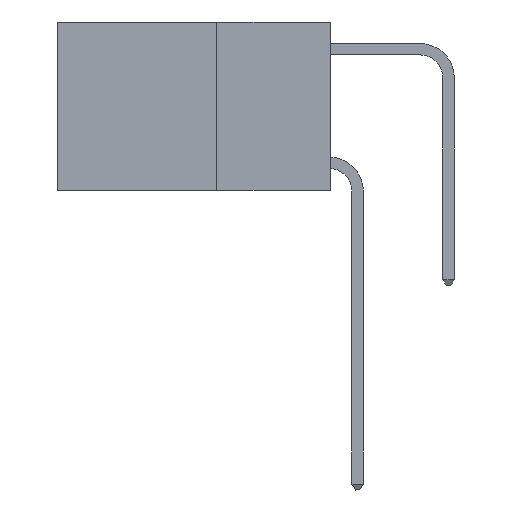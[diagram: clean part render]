
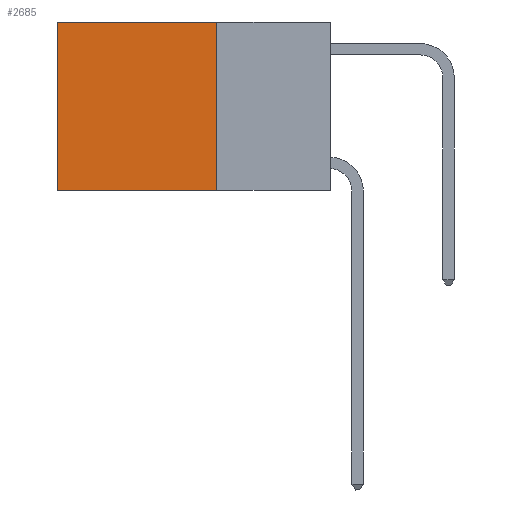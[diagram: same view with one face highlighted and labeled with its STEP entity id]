
A CAD part, left-side view. The second image highlights one B-rep face of the part: STEP entity #2685.
In plain terms, the highlighted planar face has unit normal (-1, 0, 0).
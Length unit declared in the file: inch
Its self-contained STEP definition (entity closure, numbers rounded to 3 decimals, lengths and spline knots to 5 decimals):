
#13 = DIRECTION ( 'NONE',  ( 0., 1., 0. ) ) ;
#66 = CARTESIAN_POINT ( 'NONE',  ( 0.2625, 0.25, 0. ) ) ;
#371 = CARTESIAN_POINT ( 'NONE',  ( 0.2625, 0.25, 0. ) ) ;
#1438 = VECTOR ( 'NONE', #2385, 39.37008 ) ;
#1858 = VERTEX_POINT ( 'NONE', #7121 ) ;
#2256 = EDGE_CURVE ( 'NONE', #5984, #11371, #2605, .T. ) ;
#2385 = DIRECTION ( 'NONE',  ( 0., 0., -1. ) ) ;
#2605 = LINE ( 'NONE', #66, #8923 ) ;
#2685 = ADVANCED_FACE ( 'NONE', ( #7864 ), #13582, .F. ) ;
#3142 = EDGE_LOOP ( 'NONE', ( #5998, #11830, #9302, #12167 ) ) ;
#3179 = CARTESIAN_POINT ( 'NONE',  ( 0.2625, 0.6, 0. ) ) ;
#3353 = DIRECTION ( 'NONE',  ( 0., 1., 0. ) ) ;
#4134 = AXIS2_PLACEMENT_3D ( 'NONE', #13667, #13555, #13554 ) ;
#4678 = VECTOR ( 'NONE', #10959, 39.37008 ) ;
#4725 = LINE ( 'NONE', #3179, #1438 ) ;
#5984 = VERTEX_POINT ( 'NONE', #11251 ) ;
#5998 = ORIENTED_EDGE ( 'NONE', *, *, #13751, .T. ) ;
#6033 = EDGE_CURVE ( 'NONE', #11045, #1858, #7741, .T. ) ;
#6663 = CARTESIAN_POINT ( 'NONE',  ( 0.2625, 0.25, -0.37 ) ) ;
#7121 = CARTESIAN_POINT ( 'NONE',  ( 0.2625, 0.6, -0.37 ) ) ;
#7382 = VECTOR ( 'NONE', #3353, 39.37008 ) ;
#7476 = EDGE_CURVE ( 'NONE', #5984, #11045, #11063, .T. ) ;
#7741 = LINE ( 'NONE', #8102, #7382 ) ;
#7864 = FACE_OUTER_BOUND ( 'NONE', #3142, .T. ) ;
#8102 = CARTESIAN_POINT ( 'NONE',  ( 0.2625, 0.25, -0.37 ) ) ;
#8255 = CARTESIAN_POINT ( 'NONE',  ( 0.2625, 0.6, 0. ) ) ;
#8923 = VECTOR ( 'NONE', #13, 39.37008 ) ;
#9302 = ORIENTED_EDGE ( 'NONE', *, *, #7476, .F. ) ;
#10959 = DIRECTION ( 'NONE',  ( 0., 0., -1. ) ) ;
#11045 = VERTEX_POINT ( 'NONE', #6663 ) ;
#11063 = LINE ( 'NONE', #371, #4678 ) ;
#11251 = CARTESIAN_POINT ( 'NONE',  ( 0.2625, 0.25, 0. ) ) ;
#11371 = VERTEX_POINT ( 'NONE', #8255 ) ;
#11830 = ORIENTED_EDGE ( 'NONE', *, *, #6033, .F. ) ;
#12167 = ORIENTED_EDGE ( 'NONE', *, *, #2256, .T. ) ;
#13554 = DIRECTION ( 'NONE',  ( 0., 0., -1. ) ) ;
#13555 = DIRECTION ( 'NONE',  ( 1., 0., 0. ) ) ;
#13582 = PLANE ( 'NONE',  #4134 ) ;
#13667 = CARTESIAN_POINT ( 'NONE',  ( 0.2625, 0.25, 0. ) ) ;
#13751 = EDGE_CURVE ( 'NONE', #11371, #1858, #4725, .T. ) ;
